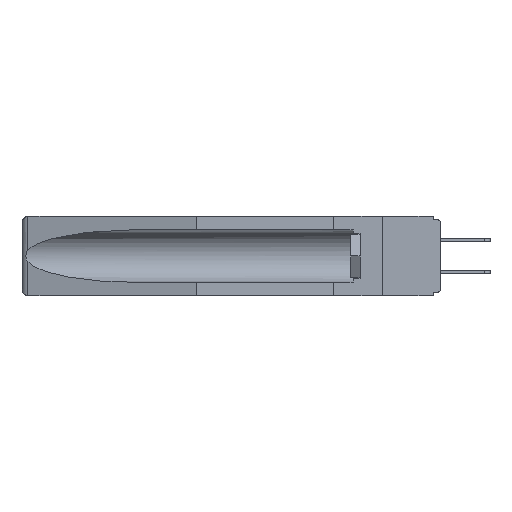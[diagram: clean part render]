
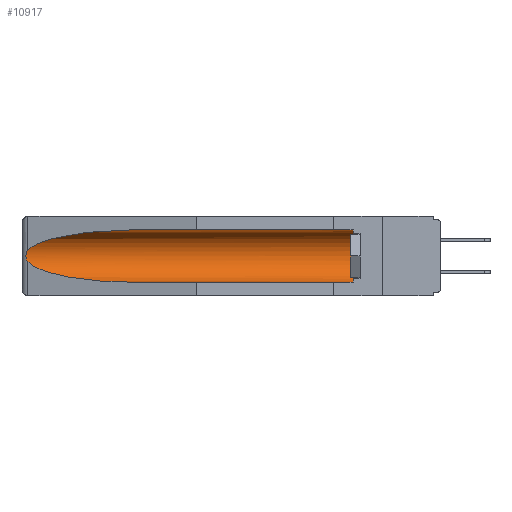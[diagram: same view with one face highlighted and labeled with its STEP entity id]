
A CAD part, left-side view. The second image highlights one B-rep face of the part: STEP entity #10917.
In plain terms, the highlighted cylindrical face has radius 2.857 mm (diameter 5.715 mm), a partial arc.
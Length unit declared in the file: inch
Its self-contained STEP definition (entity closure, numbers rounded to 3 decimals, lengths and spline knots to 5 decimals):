
#123 = CARTESIAN_POINT ( 'NONE',  ( 0.155, 1.07973, -0.059 ) ) ;
#152 = FACE_OUTER_BOUND ( 'NONE', #16795, .T. ) ;
#809 = DIRECTION ( 'NONE',  ( 0., 0., 1. ) ) ;
#856 = DIRECTION ( 'NONE',  ( 0., 1., 0. ) ) ;
#1010 = CARTESIAN_POINT ( 'NONE',  ( 0.2675, 1.53308, -0.16763 ) ) ;
#1159 = CARTESIAN_POINT ( 'NONE',  ( 0.155, 1.07973, -0.284 ) ) ;
#1226 = CARTESIAN_POINT ( 'NONE',  ( 0.26654, 1.53092, -0.15636 ) ) ;
#1626 = ORIENTED_EDGE ( 'NONE', *, *, #5943, .T. ) ;
#1770 = ORIENTED_EDGE ( 'NONE', *, *, #11163, .T. ) ;
#1990 = CARTESIAN_POINT ( 'NONE',  ( 0.21114, 1.30732, -0.059 ) ) ;
#2518 = LINE ( 'NONE', #18869, #18905 ) ;
#2533 = CIRCLE ( 'NONE', #21597, 0.1125 ) ;
#3493 = CYLINDRICAL_SURFACE ( 'NONE', #21308, 0.1125 ) ;
#3977 = LINE ( 'NONE', #19293, #9906 ) ;
#4252 = CARTESIAN_POINT ( 'NONE',  ( 0.155, 0.126, -0.1715 ) ) ;
#4345 = EDGE_CURVE ( 'NONE', #17645, #5083, #5278, .T. ) ;
#4391 = CARTESIAN_POINT ( 'NONE',  ( 0.26655, 1.53094, -0.18657 ) ) ;
#4539 = CARTESIAN_POINT ( 'NONE',  ( 0.26597, 1.5296, -0.19026 ) ) ;
#5083 = VERTEX_POINT ( 'NONE', #5742 ) ;
#5278 = B_SPLINE_CURVE_WITH_KNOTS ( 'NONE', 3,
 ( #16278, #17889, #1226, #9663, #1010, #12801, #16348, #4391, #4539, #18111 ),
 .UNSPECIFIED., .F., .F.,
 ( 4, 2, 2, 2, 4 ),
 ( 0., 0.00029, 0.00058, 0.00087, 0.00117 ),
 .UNSPECIFIED. ) ;
#5533 = VERTEX_POINT ( 'NONE', #8571 ) ;
#5742 = CARTESIAN_POINT ( 'NONE',  ( 0.26537, 1.52718, -0.19328 ) ) ;
#5840 = CARTESIAN_POINT ( 'NONE',  ( 0.155, 0.126, -0.284 ) ) ;
#5943 = EDGE_CURVE ( 'NONE', #5083, #5533, #16853, .T. ) ;
#7061 = CARTESIAN_POINT ( 'NONE',  ( 0.26537, 1.52718, -0.14972 ) ) ;
#7137 = VERTEX_POINT ( 'NONE', #123 ) ;
#7461 = DIRECTION ( 'NONE',  ( 0., 1., 0. ) ) ;
#8571 = CARTESIAN_POINT ( 'NONE',  ( 0.155, 1.07973, -0.284 ) ) ;
#8717 = CARTESIAN_POINT ( 'NONE',  ( 0.155, 0.126, -0.059 ) ) ;
#9312 = CARTESIAN_POINT ( 'NONE',  ( 0.155, -0.30754, -0.1715 ) ) ;
#9326 = ORIENTED_EDGE ( 'NONE', *, *, #11867, .T. ) ;
#9408 = EDGE_CURVE ( 'NONE', #7137, #17645, #20491, .T. ) ;
#9663 = CARTESIAN_POINT ( 'NONE',  ( 0.2673, 1.5327, -0.16383 ) ) ;
#9695 = VERTEX_POINT ( 'NONE', #8717 ) ;
#9906 = VECTOR ( 'NONE', #856, 39.37008 ) ;
#10201 = DIRECTION ( 'NONE',  ( 0., 1., 0. ) ) ;
#10395 = CARTESIAN_POINT ( 'NONE',  ( 0.155, 1.07973, -0.059 ) ) ;
#10917 = ADVANCED_FACE ( 'NONE', ( #152 ), #3493, .F. ) ;
#11101 = DIRECTION ( 'NONE',  ( 0., 0., 1. ) ) ;
#11163 = EDGE_CURVE ( 'NONE', #14115, #9695, #2533, .T. ) ;
#11817 = ORIENTED_EDGE ( 'NONE', *, *, #14215, .F. ) ;
#11867 = EDGE_CURVE ( 'NONE', #9695, #7137, #2518, .T. ) ;
#12020 = ORIENTED_EDGE ( 'NONE', *, *, #9408, .T. ) ;
#12105 = CARTESIAN_POINT ( 'NONE',  ( 0.25451, 1.48313, -0.09465 ) ) ;
#12801 = CARTESIAN_POINT ( 'NONE',  ( 0.2675, 1.53308, -0.17534 ) ) ;
#12872 = CARTESIAN_POINT ( 'NONE',  ( 0.26537, 1.52718, -0.19328 ) ) ;
#14115 = VERTEX_POINT ( 'NONE', #5840 ) ;
#14215 = EDGE_CURVE ( 'NONE', #14115, #5533, #3977, .T. ) ;
#16278 = CARTESIAN_POINT ( 'NONE',  ( 0.26537, 1.52718, -0.14972 ) ) ;
#16282 = CARTESIAN_POINT ( 'NONE',  ( 0.25451, 1.48313, -0.24835 ) ) ;
#16348 = CARTESIAN_POINT ( 'NONE',  ( 0.2673, 1.53269, -0.17917 ) ) ;
#16795 = EDGE_LOOP ( 'NONE', ( #12020, #17110, #1626, #11817, #1770, #9326 ) ) ;
#16853 =( BOUNDED_CURVE ( )  B_SPLINE_CURVE ( 3, ( #12872, #16282, #17962, #1159 ),
 .UNSPECIFIED., .F., .F. ) 
 B_SPLINE_CURVE_WITH_KNOTS ( ( 4, 4 ),
 ( 0.1948, 1.5708 ),
 .UNSPECIFIED. ) 
 CURVE ( )  GEOMETRIC_REPRESENTATION_ITEM ( )  RATIONAL_B_SPLINE_CURVE ( ( 1., 0.848, 0.848, 1. ) ) 
 REPRESENTATION_ITEM ( '' )  );
#17110 = ORIENTED_EDGE ( 'NONE', *, *, #4345, .T. ) ;
#17645 = VERTEX_POINT ( 'NONE', #7061 ) ;
#17671 = DIRECTION ( 'NONE',  ( 0., -1., 0. ) ) ;
#17889 = CARTESIAN_POINT ( 'NONE',  ( 0.26597, 1.52961, -0.15275 ) ) ;
#17962 = CARTESIAN_POINT ( 'NONE',  ( 0.21114, 1.30732, -0.284 ) ) ;
#18111 = CARTESIAN_POINT ( 'NONE',  ( 0.26537, 1.52718, -0.19328 ) ) ;
#18869 = CARTESIAN_POINT ( 'NONE',  ( 0.155, -0.30754, -0.059 ) ) ;
#18905 = VECTOR ( 'NONE', #10201, 39.37008 ) ;
#19293 = CARTESIAN_POINT ( 'NONE',  ( 0.155, -0.30754, -0.284 ) ) ;
#20450 = CARTESIAN_POINT ( 'NONE',  ( 0.26537, 1.52718, -0.14972 ) ) ;
#20491 =( BOUNDED_CURVE ( )  B_SPLINE_CURVE ( 3, ( #10395, #1990, #12105, #20450 ),
 .UNSPECIFIED., .F., .F. ) 
 B_SPLINE_CURVE_WITH_KNOTS ( ( 4, 4 ),
 ( 4.71239, 6.08839 ),
 .UNSPECIFIED. ) 
 CURVE ( )  GEOMETRIC_REPRESENTATION_ITEM ( )  RATIONAL_B_SPLINE_CURVE ( ( 1., 0.848, 0.848, 1. ) ) 
 REPRESENTATION_ITEM ( '' )  );
#21308 = AXIS2_PLACEMENT_3D ( 'NONE', #9312, #7461, #809 ) ;
#21597 = AXIS2_PLACEMENT_3D ( 'NONE', #4252, #17671, #11101 ) ;
